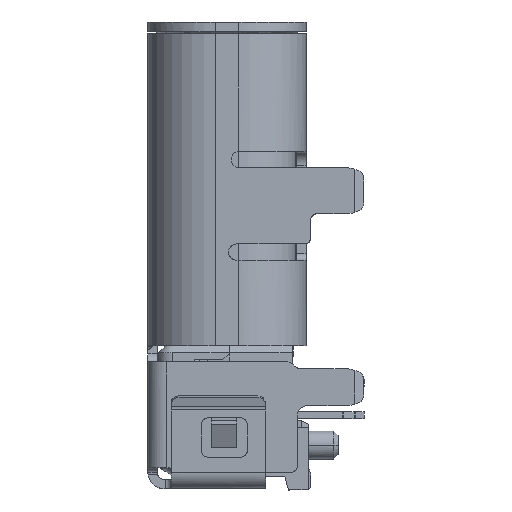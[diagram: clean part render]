
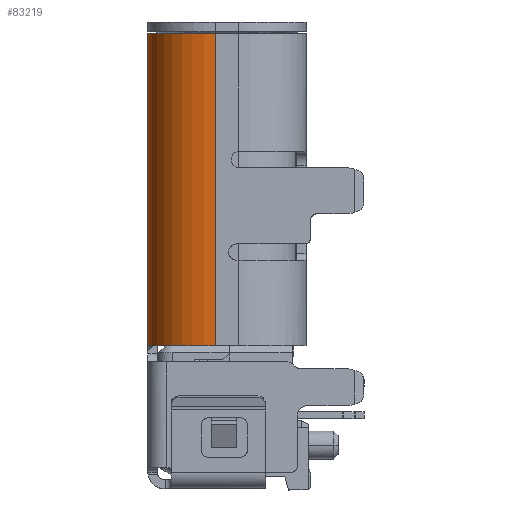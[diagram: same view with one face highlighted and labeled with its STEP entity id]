
A CAD part, left-side view. The second image highlights one B-rep face of the part: STEP entity #83219.
In plain terms, the highlighted cylindrical face has radius 1.46 mm (diameter 2.92 mm), a partial arc.
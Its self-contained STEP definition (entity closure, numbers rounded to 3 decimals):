
#227 = DIRECTION ( 'NONE',  ( 0., -1., 0. ) ) ;
#1463 = EDGE_CURVE ( 'NONE', #98196, #65739, #48490, .T. ) ;
#8866 = AXIS2_PLACEMENT_3D ( 'NONE', #19193, #19761, #100794 ) ;
#18033 = CARTESIAN_POINT ( 'NONE',  ( 21.86, -24.895, 0. ) ) ;
#18135 = AXIS2_PLACEMENT_3D ( 'NONE', #49107, #74787, #37889 ) ;
#19193 = CARTESIAN_POINT ( 'NONE',  ( 21.86, -22.755, -1.46 ) ) ;
#19372 = EDGE_LOOP ( 'NONE', ( #29338, #42609, #93004, #33903 ) ) ;
#19761 = DIRECTION ( 'NONE',  ( 0., -1., 0. ) ) ;
#22424 = VECTOR ( 'NONE', #227, 1000. ) ;
#23777 = DIRECTION ( 'NONE',  ( 0., 0., -1. ) ) ;
#24686 = EDGE_CURVE ( 'NONE', #98196, #47424, #26979, .T. ) ;
#26979 = LINE ( 'NONE', #18033, #22424 ) ;
#27071 = EDGE_CURVE ( 'NONE', #69337, #47424, #64788, .T. ) ;
#28110 = LINE ( 'NONE', #83457, #39413 ) ;
#29338 = ORIENTED_EDGE ( 'NONE', *, *, #59081, .T. ) ;
#33903 = ORIENTED_EDGE ( 'NONE', *, *, #1463, .T. ) ;
#35886 = DIRECTION ( 'NONE',  ( 0., -1., 0. ) ) ;
#37889 = DIRECTION ( 'NONE',  ( 0., 0., -1. ) ) ;
#39413 = VECTOR ( 'NONE', #35886, 1000. ) ;
#42609 = ORIENTED_EDGE ( 'NONE', *, *, #27071, .T. ) ;
#47424 = VERTEX_POINT ( 'NONE', #92793 ) ;
#48490 = CIRCLE ( 'NONE', #18135, 1.46 ) ;
#49107 = CARTESIAN_POINT ( 'NONE',  ( 21.86, -22.89, -1.46 ) ) ;
#52446 = CARTESIAN_POINT ( 'NONE',  ( 20.4, -29.64, -1.46 ) ) ;
#55093 = CARTESIAN_POINT ( 'NONE',  ( 21.86, -29.64, -1.46 ) ) ;
#56057 = CYLINDRICAL_SURFACE ( 'NONE', #8866, 1.46 ) ;
#59081 = EDGE_CURVE ( 'NONE', #65739, #69337, #28110, .T. ) ;
#64054 = CARTESIAN_POINT ( 'NONE',  ( 21.86, -22.89, 0. ) ) ;
#64437 = FACE_OUTER_BOUND ( 'NONE', #19372, .T. ) ;
#64788 = CIRCLE ( 'NONE', #87551, 1.46 ) ;
#65739 = VERTEX_POINT ( 'NONE', #75262 ) ;
#69337 = VERTEX_POINT ( 'NONE', #52446 ) ;
#74787 = DIRECTION ( 'NONE',  ( 0., -1., 0. ) ) ;
#75262 = CARTESIAN_POINT ( 'NONE',  ( 20.4, -22.89, -1.46 ) ) ;
#83219 = ADVANCED_FACE ( 'NONE', ( #64437 ), #56057, .T. ) ;
#83457 = CARTESIAN_POINT ( 'NONE',  ( 20.4, -22.755, -1.46 ) ) ;
#87551 = AXIS2_PLACEMENT_3D ( 'NONE', #55093, #105398, #23777 ) ;
#92793 = CARTESIAN_POINT ( 'NONE',  ( 21.86, -29.64, 0. ) ) ;
#93004 = ORIENTED_EDGE ( 'NONE', *, *, #24686, .F. ) ;
#98196 = VERTEX_POINT ( 'NONE', #64054 ) ;
#100794 = DIRECTION ( 'NONE',  ( 0., 0., -1. ) ) ;
#105398 = DIRECTION ( 'NONE',  ( 0., 1., 0. ) ) ;
